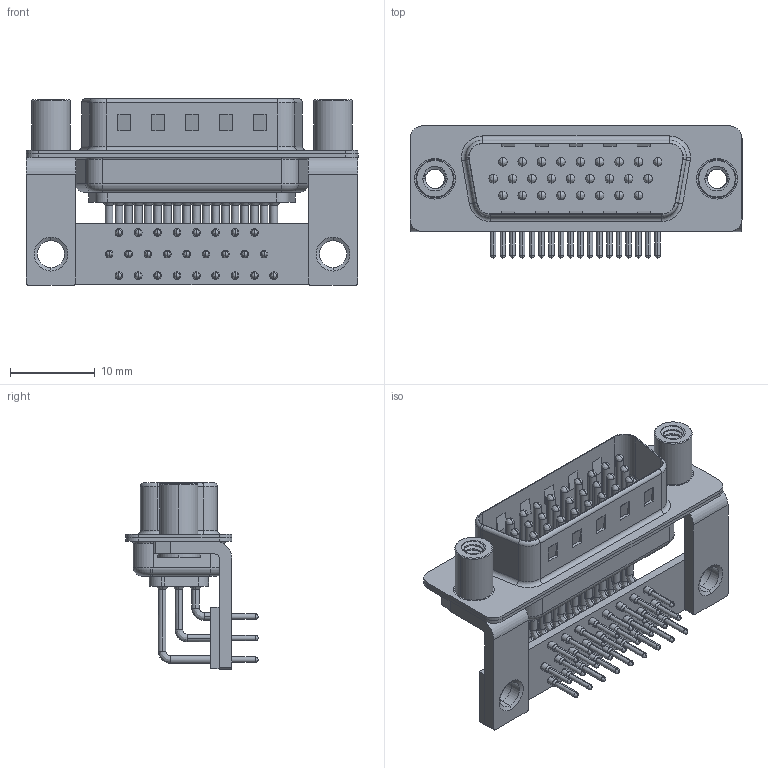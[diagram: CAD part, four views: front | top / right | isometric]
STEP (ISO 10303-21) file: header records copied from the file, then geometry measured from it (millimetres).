
FILE_DESCRIPTION (( 'STEP AP203' ), '1' );
FILE_NAME ('633-M26-363-WN6.STEP', '2018-09-27T23:21:56', ( '' ), ( '' ), 'SwSTEP 2.0', 'SolidWorks 2016', '' );
FILE_SCHEMA (( 'CONFIG_CONTROL_DESIGN' ));
Length unit declared in the file: millimetre
Products named in the file (10): 633M Shell Front_26 Contacts; 633M Shell Rear_26 Contacts; 633M 4-40 Threaded Standoff; 633M Contact Row 1; 633M Stabilizer Board_26 Contacts; 633M Contact Row 2; 633-M26-363-WN6; 633M Contact Row 3; 633M Stabilizer Bracket; 633M Housing_26 Contacts
Assembly tree (34 placements, depth 2):
  633-M26-363-WN6
    633M Housing_26 Contacts
    633M Shell Front_26 Contacts
    633M Shell Rear_26 Contacts
    633M Contact Row 1  x9
    633M Contact Row 2  x9
    633M Contact Row 3  x8
    633M Stabilizer Bracket  x2
    633M 4-40 Threaded Standoff  x2
    633M Stabilizer Board_26 Contacts
Bounding box: 39.2 x 15.6 x 22 mm (x, y, z)
Volume: 2748 mm3; surface area: 8315 mm2
Topology: 34 solids, 34 shells, 3352 faces, 9361 edges, 6090 vertices
Faces by surface type: plane 1831, cylinder 1185, bspline 162, cone 118, torus 56
Entity records: 32685 total; most frequent: CARTESIAN_POINT 7177, DIRECTION 5183, ORIENTED_EDGE 4826, EDGE_CURVE 2413, AXIS2_PLACEMENT_3D 1907, VERTEX_POINT 1571, LINE 1369, VECTOR 1369
